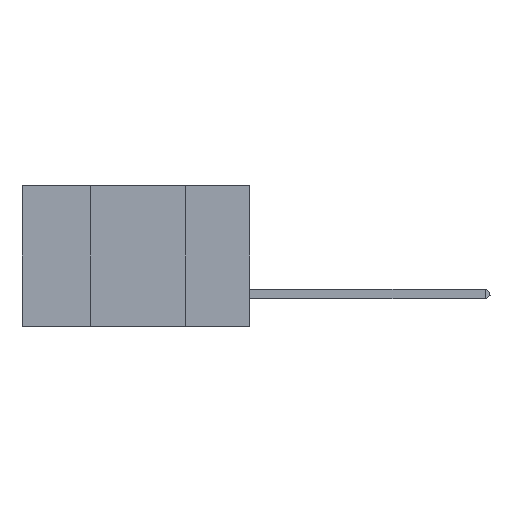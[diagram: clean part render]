
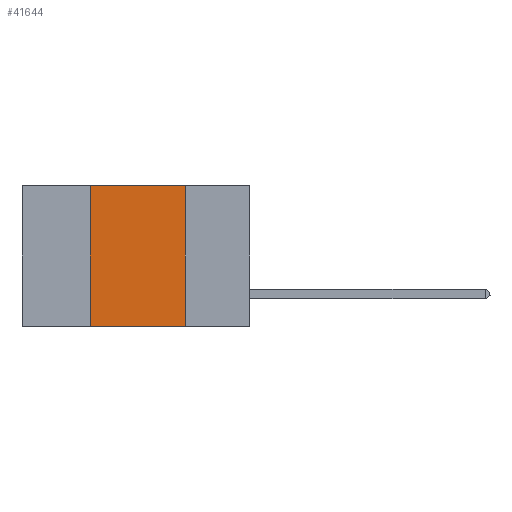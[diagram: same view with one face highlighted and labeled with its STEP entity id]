
A CAD part, left-side view. The second image highlights one B-rep face of the part: STEP entity #41644.
In plain terms, the highlighted planar face has unit normal (-1, 0, 0).
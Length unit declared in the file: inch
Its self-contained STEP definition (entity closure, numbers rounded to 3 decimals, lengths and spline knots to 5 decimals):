
#485 = LINE ( 'NONE', #34955, #44973 ) ;
#4306 = DIRECTION ( 'NONE',  ( 0., 0., -1. ) ) ;
#4440 = CARTESIAN_POINT ( 'NONE',  ( 0., 0.42, 0. ) ) ;
#5516 = DIRECTION ( 'NONE',  ( 0., -1., 0. ) ) ;
#6068 = AXIS2_PLACEMENT_3D ( 'NONE', #16383, #41907, #28202 ) ;
#6354 = DIRECTION ( 'NONE',  ( 0., 0., 1. ) ) ;
#6906 = EDGE_LOOP ( 'NONE', ( #10256, #15367, #13591, #38062 ) ) ;
#6908 = FACE_OUTER_BOUND ( 'NONE', #6906, .T. ) ;
#8096 = VECTOR ( 'NONE', #5516, 39.37008 ) ;
#10256 = ORIENTED_EDGE ( 'NONE', *, *, #28762, .F. ) ;
#10779 = VERTEX_POINT ( 'NONE', #15183 ) ;
#13079 = LINE ( 'NONE', #43323, #37625 ) ;
#13591 = ORIENTED_EDGE ( 'NONE', *, *, #43093, .F. ) ;
#13866 = VERTEX_POINT ( 'NONE', #20044 ) ;
#14400 = DIRECTION ( 'NONE',  ( 0., -1., 0. ) ) ;
#15183 = CARTESIAN_POINT ( 'NONE',  ( 0., 0.17, -0.37 ) ) ;
#15367 = ORIENTED_EDGE ( 'NONE', *, *, #38451, .F. ) ;
#16212 = CARTESIAN_POINT ( 'NONE',  ( 0., 0.6, -0.37 ) ) ;
#16383 = CARTESIAN_POINT ( 'NONE',  ( 0., 0.6, 0. ) ) ;
#20044 = CARTESIAN_POINT ( 'NONE',  ( 0., 0.17, 0. ) ) ;
#23727 = VERTEX_POINT ( 'NONE', #4440 ) ;
#25493 = VERTEX_POINT ( 'NONE', #38614 ) ;
#26181 = CARTESIAN_POINT ( 'NONE',  ( 0., 0.17, 0. ) ) ;
#28202 = DIRECTION ( 'NONE',  ( 0., 0., -1. ) ) ;
#28762 = EDGE_CURVE ( 'NONE', #13866, #10779, #45391, .T. ) ;
#31414 = PLANE ( 'NONE',  #6068 ) ;
#34802 = EDGE_CURVE ( 'NONE', #25493, #10779, #36204, .T. ) ;
#34955 = CARTESIAN_POINT ( 'NONE',  ( 0., 0.42, 0. ) ) ;
#35756 = VECTOR ( 'NONE', #4306, 39.37008 ) ;
#36204 = LINE ( 'NONE', #16212, #8096 ) ;
#37625 = VECTOR ( 'NONE', #14400, 39.37008 ) ;
#38062 = ORIENTED_EDGE ( 'NONE', *, *, #34802, .T. ) ;
#38451 = EDGE_CURVE ( 'NONE', #23727, #13866, #13079, .T. ) ;
#38614 = CARTESIAN_POINT ( 'NONE',  ( 0., 0.42, -0.37 ) ) ;
#41644 = ADVANCED_FACE ( 'NONE', ( #6908 ), #31414, .F. ) ;
#41907 = DIRECTION ( 'NONE',  ( 1., 0., 0. ) ) ;
#43093 = EDGE_CURVE ( 'NONE', #25493, #23727, #485, .T. ) ;
#43323 = CARTESIAN_POINT ( 'NONE',  ( 0., 0.6, 0. ) ) ;
#44973 = VECTOR ( 'NONE', #6354, 39.37008 ) ;
#45391 = LINE ( 'NONE', #26181, #35756 ) ;
